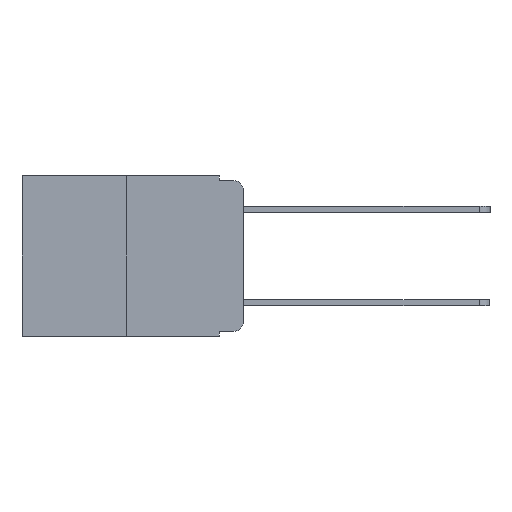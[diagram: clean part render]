
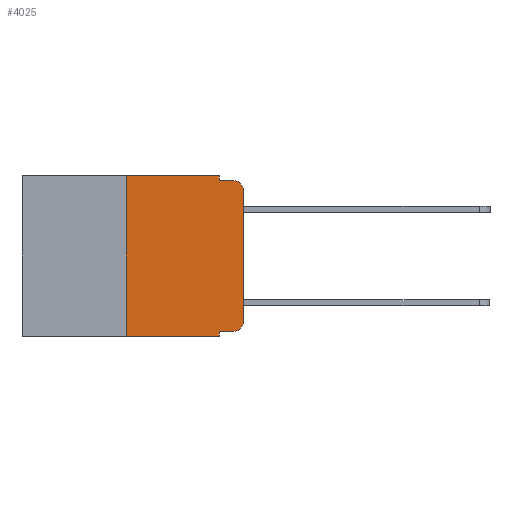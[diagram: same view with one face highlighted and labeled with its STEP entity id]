
A CAD part, left-side view. The second image highlights one B-rep face of the part: STEP entity #4025.
In plain terms, the highlighted planar face has unit normal (-1, 0, 0).
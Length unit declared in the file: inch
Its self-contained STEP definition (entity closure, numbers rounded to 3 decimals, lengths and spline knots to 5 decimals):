
#325 = EDGE_CURVE ( 'NONE', #2012, #8680, #8050, .T. ) ;
#332 = CIRCLE ( 'NONE', #1734, 0.02 ) ;
#410 = LINE ( 'NONE', #8298, #10296 ) ;
#529 = CARTESIAN_POINT ( 'NONE',  ( 0., 0.051, 0. ) ) ;
#662 = EDGE_CURVE ( 'NONE', #7593, #10522, #332, .T. ) ;
#905 = VECTOR ( 'NONE', #4574, 39.37008 ) ;
#963 = EDGE_CURVE ( 'NONE', #8057, #8680, #1989, .T. ) ;
#974 = VECTOR ( 'NONE', #6145, 39.37008 ) ;
#1099 = CARTESIAN_POINT ( 'NONE',  ( 0., 0.051, 0. ) ) ;
#1113 = FACE_OUTER_BOUND ( 'NONE', #7857, .T. ) ;
#1123 = CARTESIAN_POINT ( 'NONE',  ( 0., 0.25, -0.343 ) ) ;
#1280 = EDGE_CURVE ( 'NONE', #10400, #4842, #11901, .T. ) ;
#1352 = EDGE_CURVE ( 'NONE', #1672, #9654, #8316, .T. ) ;
#1397 = ORIENTED_EDGE ( 'NONE', *, *, #963, .T. ) ;
#1596 = ORIENTED_EDGE ( 'NONE', *, *, #662, .T. ) ;
#1626 = EDGE_CURVE ( 'NONE', #10522, #8057, #6180, .T. ) ;
#1672 = VERTEX_POINT ( 'NONE', #1123 ) ;
#1734 = AXIS2_PLACEMENT_3D ( 'NONE', #5916, #3125, #2277 ) ;
#1920 = CARTESIAN_POINT ( 'NONE',  ( 0., 0.473, 0. ) ) ;
#1989 = CIRCLE ( 'NONE', #8030, 0.02 ) ;
#2012 = VERTEX_POINT ( 'NONE', #8704 ) ;
#2050 = DIRECTION ( 'NONE',  ( 0., 0., -1. ) ) ;
#2147 = CARTESIAN_POINT ( 'NONE',  ( 0., 0.051, -0.01 ) ) ;
#2217 = ORIENTED_EDGE ( 'NONE', *, *, #8464, .T. ) ;
#2277 = DIRECTION ( 'NONE',  ( 0., 0., -1. ) ) ;
#2698 = DIRECTION ( 'NONE',  ( 0., -1., 0. ) ) ;
#2971 = CARTESIAN_POINT ( 'NONE',  ( 0., 0.02, -0.03 ) ) ;
#3014 = CARTESIAN_POINT ( 'NONE',  ( 0., 0., -0.313 ) ) ;
#3058 = DIRECTION ( 'NONE',  ( 0., 0., 1. ) ) ;
#3125 = DIRECTION ( 'NONE',  ( -1., 0., 0. ) ) ;
#3211 = CARTESIAN_POINT ( 'NONE',  ( 0., 0.051, -0.343 ) ) ;
#3219 = ORIENTED_EDGE ( 'NONE', *, *, #5945, .F. ) ;
#3450 = VECTOR ( 'NONE', #6398, 39.37008 ) ;
#3769 = ORIENTED_EDGE ( 'NONE', *, *, #325, .F. ) ;
#4023 = CARTESIAN_POINT ( 'NONE',  ( 0., 0.25, 0. ) ) ;
#4025 = ADVANCED_FACE ( 'NONE', ( #1113 ), #8525, .F. ) ;
#4110 = ORIENTED_EDGE ( 'NONE', *, *, #1280, .F. ) ;
#4197 = CARTESIAN_POINT ( 'NONE',  ( 0., 0.051, 0. ) ) ;
#4476 = DIRECTION ( 'NONE',  ( 0., -1., 0. ) ) ;
#4574 = DIRECTION ( 'NONE',  ( 0., 0., -1. ) ) ;
#4820 = CARTESIAN_POINT ( 'NONE',  ( 0., 0.02, -0.01 ) ) ;
#4842 = VERTEX_POINT ( 'NONE', #3211 ) ;
#5005 = CARTESIAN_POINT ( 'NONE',  ( 0., 0., 0. ) ) ;
#5128 = EDGE_CURVE ( 'NONE', #8958, #2012, #8840, .T. ) ;
#5219 = ORIENTED_EDGE ( 'NONE', *, *, #5128, .F. ) ;
#5226 = ORIENTED_EDGE ( 'NONE', *, *, #8707, .T. ) ;
#5245 = DIRECTION ( 'NONE',  ( -1., 0., 0. ) ) ;
#5268 = ORIENTED_EDGE ( 'NONE', *, *, #1626, .T. ) ;
#5446 = CARTESIAN_POINT ( 'NONE',  ( 0., 0.473, 0. ) ) ;
#5601 = VECTOR ( 'NONE', #3058, 39.37008 ) ;
#5822 = DIRECTION ( 'NONE',  ( 0., 0., -1. ) ) ;
#5916 = CARTESIAN_POINT ( 'NONE',  ( 0., 0.02, -0.313 ) ) ;
#5945 = EDGE_CURVE ( 'NONE', #9654, #8958, #10853, .T. ) ;
#6098 = ORIENTED_EDGE ( 'NONE', *, *, #1352, .F. ) ;
#6124 = VECTOR ( 'NONE', #7611, 39.37008 ) ;
#6145 = DIRECTION ( 'NONE',  ( 0., 0., 1. ) ) ;
#6180 = LINE ( 'NONE', #5005, #5601 ) ;
#6398 = DIRECTION ( 'NONE',  ( 0., -1., 0. ) ) ;
#6885 = DIRECTION ( 'NONE',  ( 0., 0., -1. ) ) ;
#6963 = LINE ( 'NONE', #12177, #6124 ) ;
#7593 = VERTEX_POINT ( 'NONE', #8106 ) ;
#7611 = DIRECTION ( 'NONE',  ( 0., -1., 0. ) ) ;
#7857 = EDGE_LOOP ( 'NONE', ( #5268, #1397, #3769, #5219, #3219, #6098, #5226, #4110, #2217, #1596 ) ) ;
#8030 = AXIS2_PLACEMENT_3D ( 'NONE', #2971, #5245, #2050 ) ;
#8050 = LINE ( 'NONE', #2147, #9936 ) ;
#8057 = VERTEX_POINT ( 'NONE', #11378 ) ;
#8106 = CARTESIAN_POINT ( 'NONE',  ( 0., 0.02, -0.333 ) ) ;
#8298 = CARTESIAN_POINT ( 'NONE',  ( 0., 0.051, -0.333 ) ) ;
#8316 = LINE ( 'NONE', #11634, #974 ) ;
#8391 = CARTESIAN_POINT ( 'NONE',  ( 0., 0.051, -0.333 ) ) ;
#8464 = EDGE_CURVE ( 'NONE', #10400, #7593, #410, .T. ) ;
#8525 = PLANE ( 'NONE',  #12195 ) ;
#8680 = VERTEX_POINT ( 'NONE', #4820 ) ;
#8704 = CARTESIAN_POINT ( 'NONE',  ( 0., 0.051, -0.01 ) ) ;
#8707 = EDGE_CURVE ( 'NONE', #1672, #4842, #6963, .T. ) ;
#8840 = LINE ( 'NONE', #529, #905 ) ;
#8958 = VERTEX_POINT ( 'NONE', #4197 ) ;
#9464 = VECTOR ( 'NONE', #6885, 39.37008 ) ;
#9654 = VERTEX_POINT ( 'NONE', #4023 ) ;
#9936 = VECTOR ( 'NONE', #4476, 39.37008 ) ;
#10296 = VECTOR ( 'NONE', #2698, 39.37008 ) ;
#10400 = VERTEX_POINT ( 'NONE', #8391 ) ;
#10522 = VERTEX_POINT ( 'NONE', #3014 ) ;
#10853 = LINE ( 'NONE', #5446, #3450 ) ;
#11319 = DIRECTION ( 'NONE',  ( 1., 0., 0. ) ) ;
#11378 = CARTESIAN_POINT ( 'NONE',  ( 0., 0., -0.03 ) ) ;
#11634 = CARTESIAN_POINT ( 'NONE',  ( 0., 0.25, 0. ) ) ;
#11901 = LINE ( 'NONE', #1099, #9464 ) ;
#12177 = CARTESIAN_POINT ( 'NONE',  ( 0., 0.473, -0.343 ) ) ;
#12195 = AXIS2_PLACEMENT_3D ( 'NONE', #1920, #11319, #5822 ) ;
